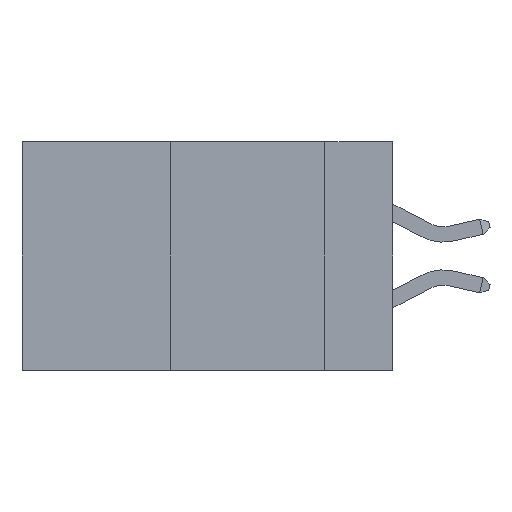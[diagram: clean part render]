
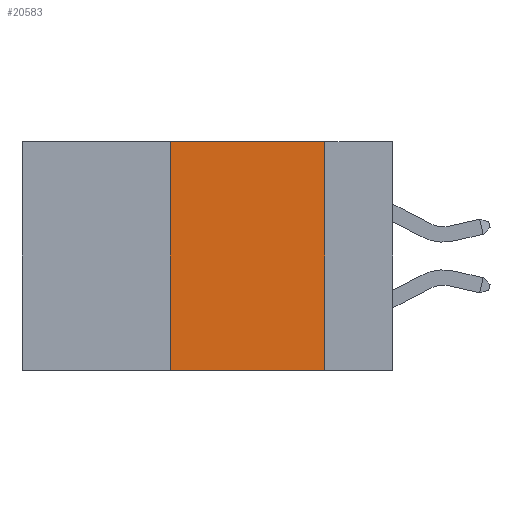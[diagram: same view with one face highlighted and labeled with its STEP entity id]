
A CAD part, left-side view. The second image highlights one B-rep face of the part: STEP entity #20583.
In plain terms, the highlighted planar face has unit normal (-1, 0, 0).
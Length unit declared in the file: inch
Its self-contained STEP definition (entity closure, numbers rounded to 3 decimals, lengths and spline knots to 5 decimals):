
#297 = VECTOR ( 'NONE', #1723, 39.37008 ) ;
#1723 = DIRECTION ( 'NONE',  ( 0., 0., 1. ) ) ;
#2285 = EDGE_LOOP ( 'NONE', ( #12313, #18668, #17470, #18111 ) ) ;
#4179 = PLANE ( 'NONE',  #32853 ) ;
#4705 = EDGE_CURVE ( 'NONE', #28785, #22676, #25033, .T. ) ;
#5080 = VECTOR ( 'NONE', #7934, 39.37008 ) ;
#6081 = VECTOR ( 'NONE', #7232, 39.37008 ) ;
#6225 = CARTESIAN_POINT ( 'NONE',  ( 0., 0.6, 0. ) ) ;
#6801 = DIRECTION ( 'NONE',  ( 0., -1., 0. ) ) ;
#7232 = DIRECTION ( 'NONE',  ( 0., -1., 0. ) ) ;
#7934 = DIRECTION ( 'NONE',  ( 0., 0., -1. ) ) ;
#8370 = VECTOR ( 'NONE', #6801, 39.37008 ) ;
#9356 = CARTESIAN_POINT ( 'NONE',  ( 0., 0.6, -0.37 ) ) ;
#9683 = CARTESIAN_POINT ( 'NONE',  ( 0., 0.11, -0.37 ) ) ;
#10167 = CARTESIAN_POINT ( 'NONE',  ( 0., 0.11, 0. ) ) ;
#12287 = CARTESIAN_POINT ( 'NONE',  ( 0., 0.36, 0. ) ) ;
#12313 = ORIENTED_EDGE ( 'NONE', *, *, #30428, .F. ) ;
#12754 = EDGE_CURVE ( 'NONE', #31594, #30422, #22141, .T. ) ;
#17122 = DIRECTION ( 'NONE',  ( 0., 0., -1. ) ) ;
#17240 = CARTESIAN_POINT ( 'NONE',  ( 0., 0.6, 0. ) ) ;
#17470 = ORIENTED_EDGE ( 'NONE', *, *, #29586, .F. ) ;
#18111 = ORIENTED_EDGE ( 'NONE', *, *, #4705, .T. ) ;
#18668 = ORIENTED_EDGE ( 'NONE', *, *, #12754, .F. ) ;
#19225 = CARTESIAN_POINT ( 'NONE',  ( 0., 0.36, -0.37 ) ) ;
#19227 = LINE ( 'NONE', #21028, #5080 ) ;
#20526 = FACE_OUTER_BOUND ( 'NONE', #2285, .T. ) ;
#20583 = ADVANCED_FACE ( 'NONE', ( #20526 ), #4179, .F. ) ;
#21028 = CARTESIAN_POINT ( 'NONE',  ( 0., 0.11, 0. ) ) ;
#22141 = LINE ( 'NONE', #6225, #8370 ) ;
#22676 = VERTEX_POINT ( 'NONE', #9683 ) ;
#24570 = CARTESIAN_POINT ( 'NONE',  ( 0., 0.36, 0. ) ) ;
#25033 = LINE ( 'NONE', #9356, #6081 ) ;
#26463 = LINE ( 'NONE', #24570, #297 ) ;
#28785 = VERTEX_POINT ( 'NONE', #19225 ) ;
#29586 = EDGE_CURVE ( 'NONE', #28785, #31594, #26463, .T. ) ;
#30422 = VERTEX_POINT ( 'NONE', #10167 ) ;
#30428 = EDGE_CURVE ( 'NONE', #30422, #22676, #19227, .T. ) ;
#31594 = VERTEX_POINT ( 'NONE', #12287 ) ;
#32527 = DIRECTION ( 'NONE',  ( 1., 0., 0. ) ) ;
#32853 = AXIS2_PLACEMENT_3D ( 'NONE', #17240, #32527, #17122 ) ;
